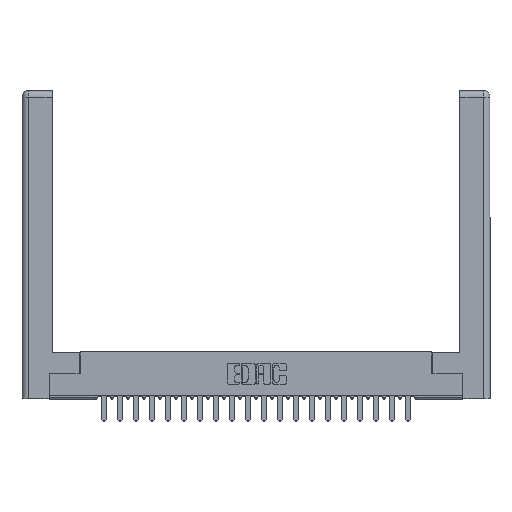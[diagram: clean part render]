
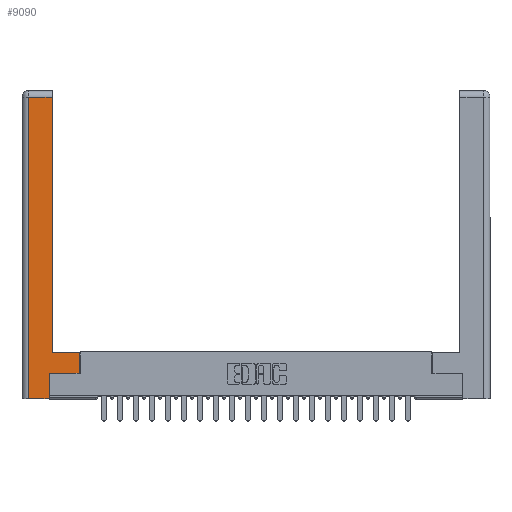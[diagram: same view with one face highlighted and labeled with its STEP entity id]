
A CAD part, top view. The second image highlights one B-rep face of the part: STEP entity #9090.
In plain terms, the highlighted planar face has unit normal (0, 0, 1).
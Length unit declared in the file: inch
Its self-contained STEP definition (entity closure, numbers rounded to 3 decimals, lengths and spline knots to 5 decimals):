
#129 = VERTEX_POINT ( 'NONE', #8316 ) ;
#818 = CARTESIAN_POINT ( 'NONE',  ( 0.265, 0., 0. ) ) ;
#930 = ORIENTED_EDGE ( 'NONE', *, *, #16718, .T. ) ;
#1740 = PLANE ( 'NONE',  #4908 ) ;
#2238 = LINE ( 'NONE', #22341, #6535 ) ;
#2283 = VECTOR ( 'NONE', #6102, 39.37008 ) ;
#2869 = CARTESIAN_POINT ( 'NONE',  ( 0.0615, 0., 0. ) ) ;
#3180 = CARTESIAN_POINT ( 'NONE',  ( 0.565, 0.45, 0. ) ) ;
#3353 = VECTOR ( 'NONE', #13150, 39.37008 ) ;
#3469 = ORIENTED_EDGE ( 'NONE', *, *, #23396, .T. ) ;
#3863 = VERTEX_POINT ( 'NONE', #20864 ) ;
#4685 = CARTESIAN_POINT ( 'NONE',  ( 0.295, 3., 0. ) ) ;
#4908 = AXIS2_PLACEMENT_3D ( 'NONE', #11371, #7704, #22337 ) ;
#5073 = VECTOR ( 'NONE', #20468, 39.37008 ) ;
#5305 = CARTESIAN_POINT ( 'NONE',  ( 0.295, 0.45, 0. ) ) ;
#5358 = LINE ( 'NONE', #24011, #5073 ) ;
#6102 = DIRECTION ( 'NONE',  ( 1., 0., 0. ) ) ;
#6535 = VECTOR ( 'NONE', #15385, 39.37008 ) ;
#7173 = DIRECTION ( 'NONE',  ( -1., 0., 0. ) ) ;
#7434 = LINE ( 'NONE', #7911, #2283 ) ;
#7704 = DIRECTION ( 'NONE',  ( 0., 0., -1. ) ) ;
#7890 = CARTESIAN_POINT ( 'NONE',  ( 0.565, 0.245, 0. ) ) ;
#7911 = CARTESIAN_POINT ( 'NONE',  ( 0.265, 0., 0. ) ) ;
#7970 = ORIENTED_EDGE ( 'NONE', *, *, #12804, .T. ) ;
#8316 = CARTESIAN_POINT ( 'NONE',  ( 0.0615, 2.94, 0. ) ) ;
#8386 = VECTOR ( 'NONE', #19922, 39.37008 ) ;
#9078 = EDGE_CURVE ( 'NONE', #14067, #3863, #12481, .T. ) ;
#9090 = ADVANCED_FACE ( 'NONE', ( #20629 ), #1740, .F. ) ;
#9101 = ORIENTED_EDGE ( 'NONE', *, *, #16712, .T. ) ;
#10112 = CARTESIAN_POINT ( 'NONE',  ( 0.0615, 0., 0. ) ) ;
#10289 = DIRECTION ( 'NONE',  ( 0., -1., 0. ) ) ;
#11371 = CARTESIAN_POINT ( 'NONE',  ( 0., 0., 0. ) ) ;
#12481 = LINE ( 'NONE', #4685, #8386 ) ;
#12804 = EDGE_CURVE ( 'NONE', #19345, #16647, #2238, .T. ) ;
#12905 = CARTESIAN_POINT ( 'NONE',  ( 0.265, 0.245, 0. ) ) ;
#13032 = ORIENTED_EDGE ( 'NONE', *, *, #21909, .T. ) ;
#13150 = DIRECTION ( 'NONE',  ( 0., 1., 0. ) ) ;
#13244 = EDGE_CURVE ( 'NONE', #16535, #13742, #7434, .T. ) ;
#13742 = VERTEX_POINT ( 'NONE', #818 ) ;
#14067 = VERTEX_POINT ( 'NONE', #5305 ) ;
#14150 = ORIENTED_EDGE ( 'NONE', *, *, #13244, .T. ) ;
#14724 = LINE ( 'NONE', #12905, #3353 ) ;
#15385 = DIRECTION ( 'NONE',  ( 0., 1., 0. ) ) ;
#15675 = LINE ( 'NONE', #7890, #23183 ) ;
#15936 = VERTEX_POINT ( 'NONE', #21783 ) ;
#16525 = VECTOR ( 'NONE', #10289, 39.37008 ) ;
#16535 = VERTEX_POINT ( 'NONE', #10112 ) ;
#16605 = EDGE_LOOP ( 'NONE', ( #18306, #930, #21499, #14150, #13032, #3469, #7970, #9101 ) ) ;
#16647 = VERTEX_POINT ( 'NONE', #3180 ) ;
#16712 = EDGE_CURVE ( 'NONE', #16647, #14067, #16791, .T. ) ;
#16718 = EDGE_CURVE ( 'NONE', #3863, #129, #5358, .T. ) ;
#16791 = LINE ( 'NONE', #20113, #17926 ) ;
#17926 = VECTOR ( 'NONE', #7173, 39.37008 ) ;
#18306 = ORIENTED_EDGE ( 'NONE', *, *, #9078, .T. ) ;
#19230 = DIRECTION ( 'NONE',  ( 1., 0., 0. ) ) ;
#19345 = VERTEX_POINT ( 'NONE', #21923 ) ;
#19922 = DIRECTION ( 'NONE',  ( 0., 1., 0. ) ) ;
#20113 = CARTESIAN_POINT ( 'NONE',  ( 0.295, 0.45, 0. ) ) ;
#20468 = DIRECTION ( 'NONE',  ( -1., 0., 0. ) ) ;
#20629 = FACE_OUTER_BOUND ( 'NONE', #16605, .T. ) ;
#20864 = CARTESIAN_POINT ( 'NONE',  ( 0.295, 2.94, 0. ) ) ;
#21391 = LINE ( 'NONE', #2869, #16525 ) ;
#21499 = ORIENTED_EDGE ( 'NONE', *, *, #22663, .T. ) ;
#21783 = CARTESIAN_POINT ( 'NONE',  ( 0.265, 0.245, 0. ) ) ;
#21909 = EDGE_CURVE ( 'NONE', #13742, #15936, #14724, .T. ) ;
#21923 = CARTESIAN_POINT ( 'NONE',  ( 0.565, 0.245, 0. ) ) ;
#22337 = DIRECTION ( 'NONE',  ( -1., 0., 0. ) ) ;
#22341 = CARTESIAN_POINT ( 'NONE',  ( 0.565, 0.45, 0. ) ) ;
#22663 = EDGE_CURVE ( 'NONE', #129, #16535, #21391, .T. ) ;
#23183 = VECTOR ( 'NONE', #19230, 39.37008 ) ;
#23396 = EDGE_CURVE ( 'NONE', #15936, #19345, #15675, .T. ) ;
#24011 = CARTESIAN_POINT ( 'NONE',  ( 0.0615, 2.94, 0. ) ) ;
